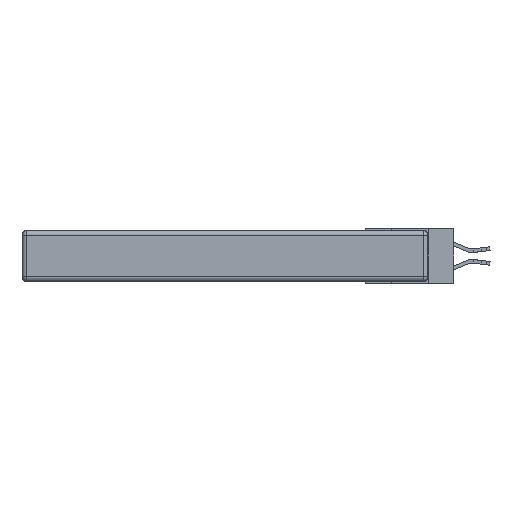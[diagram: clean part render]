
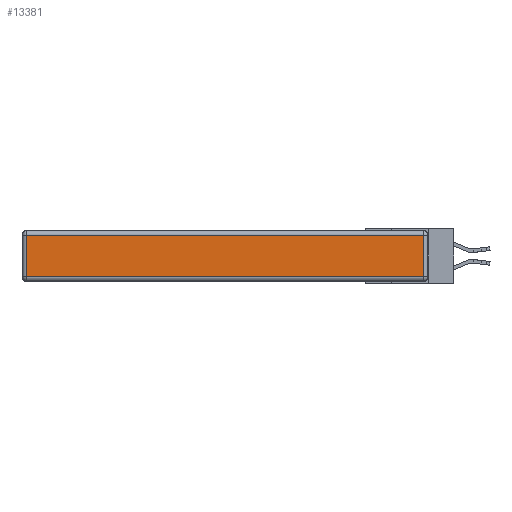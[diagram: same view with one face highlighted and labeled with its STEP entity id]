
A CAD part, left-side view. The second image highlights one B-rep face of the part: STEP entity #13381.
In plain terms, the highlighted planar face has unit normal (-1, 0, 0).
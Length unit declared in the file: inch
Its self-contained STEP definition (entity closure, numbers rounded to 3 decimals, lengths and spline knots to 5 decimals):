
#82 = AXIS2_PLACEMENT_3D ( 'NONE', #15950, #8943, #7156 ) ;
#362 = VECTOR ( 'NONE', #6589, 39.37008 ) ;
#384 = ORIENTED_EDGE ( 'NONE', *, *, #8750, .T. ) ;
#644 = EDGE_CURVE ( 'NONE', #2022, #18304, #15220, .T. ) ;
#1261 = EDGE_CURVE ( 'NONE', #11911, #2022, #11732, .T. ) ;
#1841 = EDGE_CURVE ( 'NONE', #18304, #10350, #11209, .T. ) ;
#2022 = VERTEX_POINT ( 'NONE', #10609 ) ;
#2363 = CARTESIAN_POINT ( 'NONE',  ( 0., 0.03, -0.313 ) ) ;
#6126 = PLANE ( 'NONE',  #82 ) ;
#6589 = DIRECTION ( 'NONE',  ( 0., 0., -1. ) ) ;
#7156 = DIRECTION ( 'NONE',  ( 0., 0., 1. ) ) ;
#7246 = CARTESIAN_POINT ( 'NONE',  ( 0., 0., -0.313 ) ) ;
#8750 = EDGE_CURVE ( 'NONE', #10350, #11911, #10942, .T. ) ;
#8941 = VECTOR ( 'NONE', #14483, 39.37008 ) ;
#8943 = DIRECTION ( 'NONE',  ( -1., 0., 0. ) ) ;
#9303 = DIRECTION ( 'NONE',  ( 0., 1., 0. ) ) ;
#9618 = CARTESIAN_POINT ( 'NONE',  ( 0., 2.72, -0.313 ) ) ;
#10350 = VERTEX_POINT ( 'NONE', #9618 ) ;
#10609 = CARTESIAN_POINT ( 'NONE',  ( 0., 0.03, -0.03 ) ) ;
#10827 = CARTESIAN_POINT ( 'NONE',  ( 0., 2.72, -0.343 ) ) ;
#10942 = LINE ( 'NONE', #7246, #8941 ) ;
#11209 = LINE ( 'NONE', #10827, #362 ) ;
#11537 = ORIENTED_EDGE ( 'NONE', *, *, #644, .T. ) ;
#11732 = LINE ( 'NONE', #13709, #13252 ) ;
#11811 = ORIENTED_EDGE ( 'NONE', *, *, #1841, .T. ) ;
#11911 = VERTEX_POINT ( 'NONE', #2363 ) ;
#13056 = VECTOR ( 'NONE', #9303, 39.37008 ) ;
#13252 = VECTOR ( 'NONE', #15338, 39.37008 ) ;
#13329 = CARTESIAN_POINT ( 'NONE',  ( 0., 2.72, -0.03 ) ) ;
#13381 = ADVANCED_FACE ( 'NONE', ( #17853 ), #6126, .T. ) ;
#13709 = CARTESIAN_POINT ( 'NONE',  ( 0., 0.03, -0.343 ) ) ;
#14483 = DIRECTION ( 'NONE',  ( 0., -1., 0. ) ) ;
#14493 = EDGE_LOOP ( 'NONE', ( #384, #17600, #11537, #11811 ) ) ;
#15220 = LINE ( 'NONE', #17797, #13056 ) ;
#15338 = DIRECTION ( 'NONE',  ( 0., 0., 1. ) ) ;
#15950 = CARTESIAN_POINT ( 'NONE',  ( 0., 0., -0.343 ) ) ;
#17600 = ORIENTED_EDGE ( 'NONE', *, *, #1261, .T. ) ;
#17797 = CARTESIAN_POINT ( 'NONE',  ( 0., 2.75, -0.03 ) ) ;
#17853 = FACE_OUTER_BOUND ( 'NONE', #14493, .T. ) ;
#18304 = VERTEX_POINT ( 'NONE', #13329 ) ;
